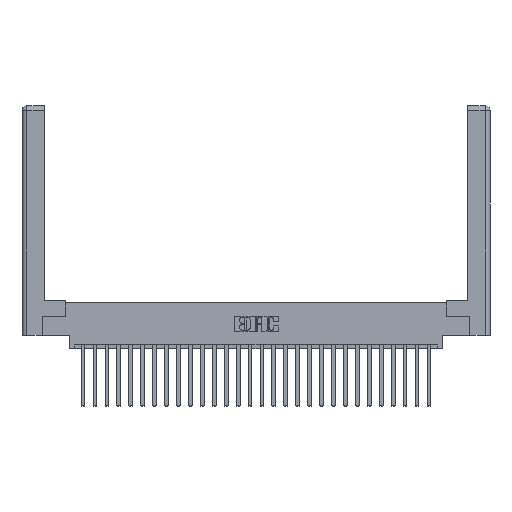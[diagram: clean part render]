
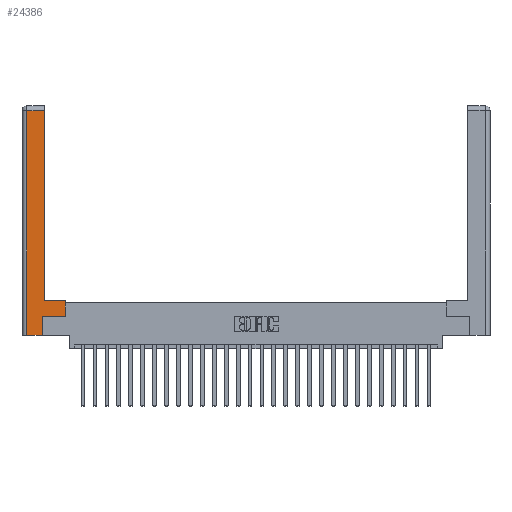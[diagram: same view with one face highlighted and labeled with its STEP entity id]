
A CAD part, top view. The second image highlights one B-rep face of the part: STEP entity #24386.
In plain terms, the highlighted planar face has unit normal (0, 0, 1).
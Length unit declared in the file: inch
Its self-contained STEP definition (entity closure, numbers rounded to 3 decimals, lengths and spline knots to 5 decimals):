
#240 = DIRECTION ( 'NONE',  ( 0., 1., 0. ) ) ;
#298 = VECTOR ( 'NONE', #18646, 39.37008 ) ;
#931 = DIRECTION ( 'NONE',  ( 1., 0., 0. ) ) ;
#1368 = CARTESIAN_POINT ( 'NONE',  ( 0.565, 0.45, 0. ) ) ;
#1735 = ORIENTED_EDGE ( 'NONE', *, *, #14715, .T. ) ;
#1802 = VECTOR ( 'NONE', #11594, 39.37008 ) ;
#1905 = VECTOR ( 'NONE', #10795, 39.37008 ) ;
#1910 = ORIENTED_EDGE ( 'NONE', *, *, #7520, .T. ) ;
#2002 = FACE_OUTER_BOUND ( 'NONE', #26837, .T. ) ;
#2130 = CARTESIAN_POINT ( 'NONE',  ( 0.565, 0.245, 0. ) ) ;
#2876 = VERTEX_POINT ( 'NONE', #8519 ) ;
#3299 = CARTESIAN_POINT ( 'NONE',  ( 0.265, 0.245, 0. ) ) ;
#3373 = EDGE_CURVE ( 'NONE', #2876, #17011, #15740, .T. ) ;
#4674 = CARTESIAN_POINT ( 'NONE',  ( 0.565, 0.45, 0. ) ) ;
#4701 = CARTESIAN_POINT ( 'NONE',  ( 0.295, 2.94, 0. ) ) ;
#5375 = ORIENTED_EDGE ( 'NONE', *, *, #16400, .T. ) ;
#5560 = VERTEX_POINT ( 'NONE', #26080 ) ;
#6260 = DIRECTION ( 'NONE',  ( -1., 0., 0. ) ) ;
#6381 = ORIENTED_EDGE ( 'NONE', *, *, #3373, .T. ) ;
#6559 = EDGE_CURVE ( 'NONE', #12430, #17313, #14206, .T. ) ;
#6704 = CARTESIAN_POINT ( 'NONE',  ( 0.0615, 0., 0. ) ) ;
#6943 = VECTOR ( 'NONE', #10863, 39.37008 ) ;
#7245 = CARTESIAN_POINT ( 'NONE',  ( 0.265, 0., 0. ) ) ;
#7520 = EDGE_CURVE ( 'NONE', #17313, #13585, #7547, .T. ) ;
#7547 = LINE ( 'NONE', #6704, #1905 ) ;
#8206 = CARTESIAN_POINT ( 'NONE',  ( 0., 0., 0. ) ) ;
#8290 = CARTESIAN_POINT ( 'NONE',  ( 0.265, 0.245, 0. ) ) ;
#8360 = LINE ( 'NONE', #7245, #20663 ) ;
#8519 = CARTESIAN_POINT ( 'NONE',  ( 0.265, 0., 0. ) ) ;
#8642 = CARTESIAN_POINT ( 'NONE',  ( 0.0615, 0., 0. ) ) ;
#8780 = DIRECTION ( 'NONE',  ( -1., 0., 0. ) ) ;
#8789 = VECTOR ( 'NONE', #23401, 39.37008 ) ;
#8997 = VECTOR ( 'NONE', #8780, 39.37008 ) ;
#9507 = EDGE_CURVE ( 'NONE', #5560, #21234, #11862, .T. ) ;
#9911 = LINE ( 'NONE', #2130, #6943 ) ;
#10520 = CARTESIAN_POINT ( 'NONE',  ( 0.0615, 2.94, 0. ) ) ;
#10683 = ORIENTED_EDGE ( 'NONE', *, *, #9507, .T. ) ;
#10723 = CARTESIAN_POINT ( 'NONE',  ( 0.0615, 2.94, 0. ) ) ;
#10795 = DIRECTION ( 'NONE',  ( 0., -1., 0. ) ) ;
#10863 = DIRECTION ( 'NONE',  ( 1., 0., 0. ) ) ;
#10993 = LINE ( 'NONE', #15066, #8997 ) ;
#11594 = DIRECTION ( 'NONE',  ( 0., 1., 0. ) ) ;
#11862 = LINE ( 'NONE', #4674, #14819 ) ;
#11903 = AXIS2_PLACEMENT_3D ( 'NONE', #8206, #23217, #6260 ) ;
#12430 = VERTEX_POINT ( 'NONE', #4701 ) ;
#12796 = LINE ( 'NONE', #24557, #1802 ) ;
#13585 = VERTEX_POINT ( 'NONE', #8642 ) ;
#14206 = LINE ( 'NONE', #10520, #298 ) ;
#14715 = EDGE_CURVE ( 'NONE', #21014, #12430, #12796, .T. ) ;
#14819 = VECTOR ( 'NONE', #240, 39.37008 ) ;
#15066 = CARTESIAN_POINT ( 'NONE',  ( 0.295, 0.45, 0. ) ) ;
#15740 = LINE ( 'NONE', #8290, #8789 ) ;
#16400 = EDGE_CURVE ( 'NONE', #13585, #2876, #8360, .T. ) ;
#16719 = PLANE ( 'NONE',  #11903 ) ;
#16743 = ORIENTED_EDGE ( 'NONE', *, *, #6559, .T. ) ;
#17011 = VERTEX_POINT ( 'NONE', #3299 ) ;
#17313 = VERTEX_POINT ( 'NONE', #10723 ) ;
#18028 = ORIENTED_EDGE ( 'NONE', *, *, #19349, .T. ) ;
#18175 = EDGE_CURVE ( 'NONE', #21234, #21014, #10993, .T. ) ;
#18646 = DIRECTION ( 'NONE',  ( -1., 0., 0. ) ) ;
#19349 = EDGE_CURVE ( 'NONE', #17011, #5560, #9911, .T. ) ;
#19400 = CARTESIAN_POINT ( 'NONE',  ( 0.295, 0.45, 0. ) ) ;
#20663 = VECTOR ( 'NONE', #931, 39.37008 ) ;
#21014 = VERTEX_POINT ( 'NONE', #19400 ) ;
#21234 = VERTEX_POINT ( 'NONE', #1368 ) ;
#22980 = ORIENTED_EDGE ( 'NONE', *, *, #18175, .T. ) ;
#23217 = DIRECTION ( 'NONE',  ( 0., 0., -1. ) ) ;
#23401 = DIRECTION ( 'NONE',  ( 0., 1., 0. ) ) ;
#24386 = ADVANCED_FACE ( 'NONE', ( #2002 ), #16719, .F. ) ;
#24557 = CARTESIAN_POINT ( 'NONE',  ( 0.295, 3., 0. ) ) ;
#26080 = CARTESIAN_POINT ( 'NONE',  ( 0.565, 0.245, 0. ) ) ;
#26837 = EDGE_LOOP ( 'NONE', ( #1735, #16743, #1910, #5375, #6381, #18028, #10683, #22980 ) ) ;
